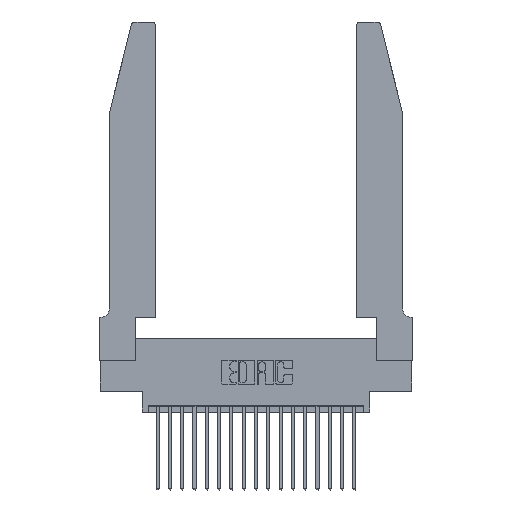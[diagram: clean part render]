
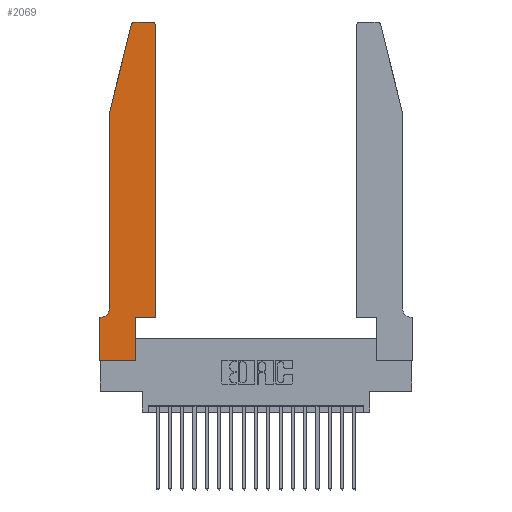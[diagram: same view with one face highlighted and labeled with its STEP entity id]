
A CAD part, top view. The second image highlights one B-rep face of the part: STEP entity #2069.
In plain terms, the highlighted planar face has unit normal (0, 0, 1).
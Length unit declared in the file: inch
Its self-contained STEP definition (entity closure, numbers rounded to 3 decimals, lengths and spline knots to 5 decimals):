
#40 = LINE ( 'NONE', #7164, #5552 ) ;
#151 = DIRECTION ( 'NONE',  ( 1., 0., 0. ) ) ;
#385 = VERTEX_POINT ( 'NONE', #2496 ) ;
#589 = ORIENTED_EDGE ( 'NONE', *, *, #17147, .T. ) ;
#862 = ORIENTED_EDGE ( 'NONE', *, *, #16073, .T. ) ;
#939 = EDGE_CURVE ( 'NONE', #15829, #18951, #40, .T. ) ;
#970 = ORIENTED_EDGE ( 'NONE', *, *, #14826, .T. ) ;
#1169 = CARTESIAN_POINT ( 'NONE',  ( 0.2865, 0., 0.37 ) ) ;
#1348 = VERTEX_POINT ( 'NONE', #3117 ) ;
#1467 = CARTESIAN_POINT ( 'NONE',  ( 0.0755, 0.42, 0.37 ) ) ;
#1588 = EDGE_CURVE ( 'NONE', #5613, #6156, #2911, .T. ) ;
#2069 = ADVANCED_FACE ( 'NONE', ( #4467 ), #15139, .T. ) ;
#2246 = DIRECTION ( 'NONE',  ( 1., 0., 0. ) ) ;
#2274 = VECTOR ( 'NONE', #3828, 39.37008 ) ;
#2281 = ORIENTED_EDGE ( 'NONE', *, *, #3132, .T. ) ;
#2418 = DIRECTION ( 'NONE',  ( 1., 0., 0. ) ) ;
#2496 = CARTESIAN_POINT ( 'NONE',  ( 0.284, 2.75, 0.37 ) ) ;
#2911 = LINE ( 'NONE', #3832, #15153 ) ;
#3102 = CARTESIAN_POINT ( 'NONE',  ( 0.2865, 0.35, 0.37 ) ) ;
#3117 = CARTESIAN_POINT ( 'NONE',  ( 0.4505, 2.72, 0.37 ) ) ;
#3132 = EDGE_CURVE ( 'NONE', #8111, #385, #5715, .T. ) ;
#3683 = CARTESIAN_POINT ( 'NONE',  ( 0.0755, 0.35, 0.37 ) ) ;
#3828 = DIRECTION ( 'NONE',  ( -1., 0., 0. ) ) ;
#3832 = CARTESIAN_POINT ( 'NONE',  ( 0.0755, 2., 0.37 ) ) ;
#3927 = LINE ( 'NONE', #8100, #15897 ) ;
#4138 = DIRECTION ( 'NONE',  ( 0., 0., 1. ) ) ;
#4467 = FACE_OUTER_BOUND ( 'NONE', #8371, .T. ) ;
#4714 = DIRECTION ( 'NONE',  ( -1., 0., 0. ) ) ;
#5072 = VECTOR ( 'NONE', #15067, 39.37008 ) ;
#5083 = CARTESIAN_POINT ( 'NONE',  ( 0.4505, 0.35, 0.37 ) ) ;
#5245 = DIRECTION ( 'NONE',  ( 1., 0., 0. ) ) ;
#5530 = VECTOR ( 'NONE', #16709, 39.37008 ) ;
#5552 = VECTOR ( 'NONE', #2418, 39.37008 ) ;
#5613 = VERTEX_POINT ( 'NONE', #8022 ) ;
#5715 = LINE ( 'NONE', #7923, #7012 ) ;
#6156 = VERTEX_POINT ( 'NONE', #1467 ) ;
#6238 = VERTEX_POINT ( 'NONE', #13060 ) ;
#6637 = ORIENTED_EDGE ( 'NONE', *, *, #939, .T. ) ;
#6846 = CARTESIAN_POINT ( 'NONE',  ( 0., 0.35, 0.37 ) ) ;
#6876 = CARTESIAN_POINT ( 'NONE',  ( 0., 0.35, 0.37 ) ) ;
#7012 = VECTOR ( 'NONE', #4714, 39.37008 ) ;
#7106 = ORIENTED_EDGE ( 'NONE', *, *, #8265, .T. ) ;
#7164 = CARTESIAN_POINT ( 'NONE',  ( 0., 0., 0.37 ) ) ;
#7373 = VERTEX_POINT ( 'NONE', #16597 ) ;
#7558 = CIRCLE ( 'NONE', #21236, 0.07 ) ;
#7849 = VECTOR ( 'NONE', #151, 39.37008 ) ;
#7923 = CARTESIAN_POINT ( 'NONE',  ( 0.2605, 2.75, 0.37 ) ) ;
#7926 = EDGE_CURVE ( 'NONE', #19288, #7373, #17979, .T. ) ;
#7931 = CARTESIAN_POINT ( 'NONE',  ( 0.25487, 2.72718, 0.37 ) ) ;
#8022 = CARTESIAN_POINT ( 'NONE',  ( 0.0755, 2., 0.37 ) ) ;
#8100 = CARTESIAN_POINT ( 'NONE',  ( 0., 0., 0.37 ) ) ;
#8111 = VERTEX_POINT ( 'NONE', #17277 ) ;
#8193 = ORIENTED_EDGE ( 'NONE', *, *, #10140, .T. ) ;
#8232 = ORIENTED_EDGE ( 'NONE', *, *, #15702, .T. ) ;
#8265 = EDGE_CURVE ( 'NONE', #11154, #15829, #3927, .T. ) ;
#8371 = EDGE_LOOP ( 'NONE', ( #2281, #8193, #970, #20081, #8232, #589, #7106, #6637, #21484, #10470, #12792, #862 ) ) ;
#8585 = CARTESIAN_POINT ( 'NONE',  ( 0.2865, 0.35, 0.37 ) ) ;
#9642 = CARTESIAN_POINT ( 'NONE',  ( 0.0055, 0.42, 0.37 ) ) ;
#10140 = EDGE_CURVE ( 'NONE', #385, #20579, #12446, .T. ) ;
#10470 = ORIENTED_EDGE ( 'NONE', *, *, #7926, .T. ) ;
#10544 = DIRECTION ( 'NONE',  ( -0.239, -0.971, 0. ) ) ;
#11130 = AXIS2_PLACEMENT_3D ( 'NONE', #15780, #4138, #19140 ) ;
#11154 = VERTEX_POINT ( 'NONE', #6876 ) ;
#11484 = DIRECTION ( 'NONE',  ( 0., -1., 0. ) ) ;
#11668 = EDGE_CURVE ( 'NONE', #18951, #19288, #18642, .T. ) ;
#11755 = CARTESIAN_POINT ( 'NONE',  ( 0., 0., 0.37 ) ) ;
#11959 = DIRECTION ( 'NONE',  ( 0., 0., 1. ) ) ;
#12205 = DIRECTION ( 'NONE',  ( 0., -1., 0. ) ) ;
#12446 = CIRCLE ( 'NONE', #11130, 0.03 ) ;
#12792 = ORIENTED_EDGE ( 'NONE', *, *, #12910, .T. ) ;
#12910 = EDGE_CURVE ( 'NONE', #7373, #1348, #18823, .T. ) ;
#13060 = CARTESIAN_POINT ( 'NONE',  ( 0.0055, 0.35, 0.37 ) ) ;
#14653 = DIRECTION ( 'NONE',  ( -1., 0., 0. ) ) ;
#14826 = EDGE_CURVE ( 'NONE', #20579, #5613, #14886, .T. ) ;
#14886 = LINE ( 'NONE', #20741, #18812 ) ;
#15067 = DIRECTION ( 'NONE',  ( 0., 1., 0. ) ) ;
#15139 = PLANE ( 'NONE',  #20667 ) ;
#15153 = VECTOR ( 'NONE', #12205, 39.37008 ) ;
#15501 = CARTESIAN_POINT ( 'NONE',  ( 0.4205, 2.72, 0.37 ) ) ;
#15702 = EDGE_CURVE ( 'NONE', #6156, #6238, #7558, .T. ) ;
#15780 = CARTESIAN_POINT ( 'NONE',  ( 0.284, 2.72, 0.37 ) ) ;
#15829 = VERTEX_POINT ( 'NONE', #11755 ) ;
#15897 = VECTOR ( 'NONE', #11484, 39.37008 ) ;
#16073 = EDGE_CURVE ( 'NONE', #1348, #8111, #20821, .T. ) ;
#16597 = CARTESIAN_POINT ( 'NONE',  ( 0.4505, 0.35, 0.37 ) ) ;
#16709 = DIRECTION ( 'NONE',  ( 0., 1., 0. ) ) ;
#17147 = EDGE_CURVE ( 'NONE', #6238, #11154, #18424, .T. ) ;
#17277 = CARTESIAN_POINT ( 'NONE',  ( 0.4205, 2.75, 0.37 ) ) ;
#17858 = AXIS2_PLACEMENT_3D ( 'NONE', #15501, #18861, #2246 ) ;
#17979 = LINE ( 'NONE', #18625, #7849 ) ;
#18424 = LINE ( 'NONE', #3683, #2274 ) ;
#18625 = CARTESIAN_POINT ( 'NONE',  ( 0.4505, 0.35, 0.37 ) ) ;
#18642 = LINE ( 'NONE', #8585, #5072 ) ;
#18812 = VECTOR ( 'NONE', #10544, 39.37008 ) ;
#18823 = LINE ( 'NONE', #5083, #5530 ) ;
#18861 = DIRECTION ( 'NONE',  ( 0., 0., 1. ) ) ;
#18951 = VERTEX_POINT ( 'NONE', #1169 ) ;
#19140 = DIRECTION ( 'NONE',  ( 1., 0., 0. ) ) ;
#19288 = VERTEX_POINT ( 'NONE', #3102 ) ;
#20081 = ORIENTED_EDGE ( 'NONE', *, *, #1588, .T. ) ;
#20579 = VERTEX_POINT ( 'NONE', #7931 ) ;
#20667 = AXIS2_PLACEMENT_3D ( 'NONE', #6846, #11959, #5245 ) ;
#20741 = CARTESIAN_POINT ( 'NONE',  ( 0.0755, 2., 0.37 ) ) ;
#20821 = CIRCLE ( 'NONE', #17858, 0.03 ) ;
#21236 = AXIS2_PLACEMENT_3D ( 'NONE', #9642, #21320, #14653 ) ;
#21320 = DIRECTION ( 'NONE',  ( 0., 0., -1. ) ) ;
#21484 = ORIENTED_EDGE ( 'NONE', *, *, #11668, .T. ) ;
